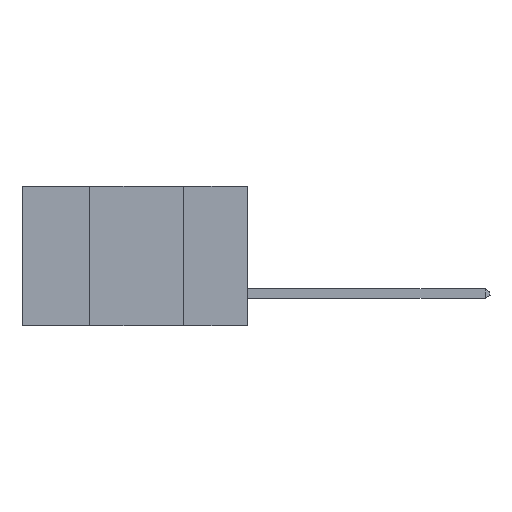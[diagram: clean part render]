
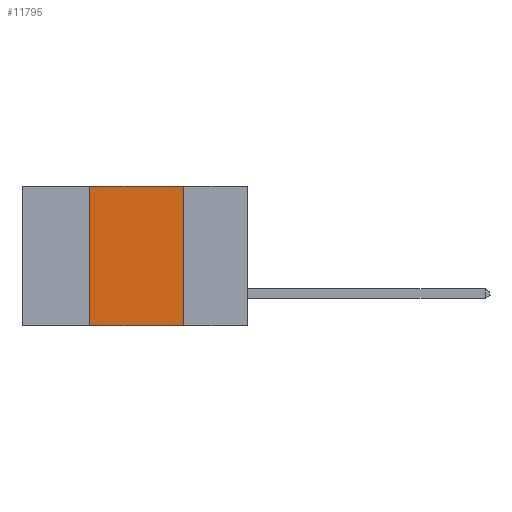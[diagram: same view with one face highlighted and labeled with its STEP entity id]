
A CAD part, left-side view. The second image highlights one B-rep face of the part: STEP entity #11795.
In plain terms, the highlighted planar face has unit normal (-1, 0, 0).
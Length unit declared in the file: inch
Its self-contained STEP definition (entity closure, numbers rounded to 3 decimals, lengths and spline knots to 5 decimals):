
#91 = LINE ( 'NONE', #10018, #3240 ) ;
#334 = AXIS2_PLACEMENT_3D ( 'NONE', #12283, #6617, #4668 ) ;
#627 = CARTESIAN_POINT ( 'NONE',  ( 0., 0.6, -0.37 ) ) ;
#649 = EDGE_CURVE ( 'NONE', #4167, #10020, #9250, .T. ) ;
#864 = LINE ( 'NONE', #11887, #9947 ) ;
#1188 = ORIENTED_EDGE ( 'NONE', *, *, #5890, .F. ) ;
#1301 = EDGE_LOOP ( 'NONE', ( #1188, #7056, #1825, #10364 ) ) ;
#1775 = PLANE ( 'NONE',  #334 ) ;
#1825 = ORIENTED_EDGE ( 'NONE', *, *, #5340, .F. ) ;
#2562 = VECTOR ( 'NONE', #3377, 39.37008 ) ;
#3240 = VECTOR ( 'NONE', #11738, 39.37008 ) ;
#3377 = DIRECTION ( 'NONE',  ( 0., -1., 0. ) ) ;
#3458 = CARTESIAN_POINT ( 'NONE',  ( 0., 0.17, 0. ) ) ;
#4167 = VERTEX_POINT ( 'NONE', #6207 ) ;
#4668 = DIRECTION ( 'NONE',  ( 0., 0., -1. ) ) ;
#5340 = EDGE_CURVE ( 'NONE', #10689, #4167, #864, .T. ) ;
#5492 = DIRECTION ( 'NONE',  ( 0., -1., 0. ) ) ;
#5890 = EDGE_CURVE ( 'NONE', #10020, #6263, #91, .T. ) ;
#6207 = CARTESIAN_POINT ( 'NONE',  ( 0., 0.42, 0. ) ) ;
#6263 = VERTEX_POINT ( 'NONE', #8913 ) ;
#6617 = DIRECTION ( 'NONE',  ( 1., 0., 0. ) ) ;
#7056 = ORIENTED_EDGE ( 'NONE', *, *, #649, .F. ) ;
#7590 = CARTESIAN_POINT ( 'NONE',  ( 0., 0.42, -0.37 ) ) ;
#8913 = CARTESIAN_POINT ( 'NONE',  ( 0., 0.17, -0.37 ) ) ;
#8921 = DIRECTION ( 'NONE',  ( 0., 0., 1. ) ) ;
#8989 = CARTESIAN_POINT ( 'NONE',  ( 0., 0.6, 0. ) ) ;
#9175 = FACE_OUTER_BOUND ( 'NONE', #1301, .T. ) ;
#9250 = LINE ( 'NONE', #8989, #2562 ) ;
#9458 = EDGE_CURVE ( 'NONE', #10689, #6263, #12157, .T. ) ;
#9947 = VECTOR ( 'NONE', #8921, 39.37008 ) ;
#10018 = CARTESIAN_POINT ( 'NONE',  ( 0., 0.17, 0. ) ) ;
#10020 = VERTEX_POINT ( 'NONE', #3458 ) ;
#10364 = ORIENTED_EDGE ( 'NONE', *, *, #9458, .T. ) ;
#10689 = VERTEX_POINT ( 'NONE', #7590 ) ;
#11135 = VECTOR ( 'NONE', #5492, 39.37008 ) ;
#11738 = DIRECTION ( 'NONE',  ( 0., 0., -1. ) ) ;
#11795 = ADVANCED_FACE ( 'NONE', ( #9175 ), #1775, .F. ) ;
#11887 = CARTESIAN_POINT ( 'NONE',  ( 0., 0.42, 0. ) ) ;
#12157 = LINE ( 'NONE', #627, #11135 ) ;
#12283 = CARTESIAN_POINT ( 'NONE',  ( 0., 0.6, 0. ) ) ;
